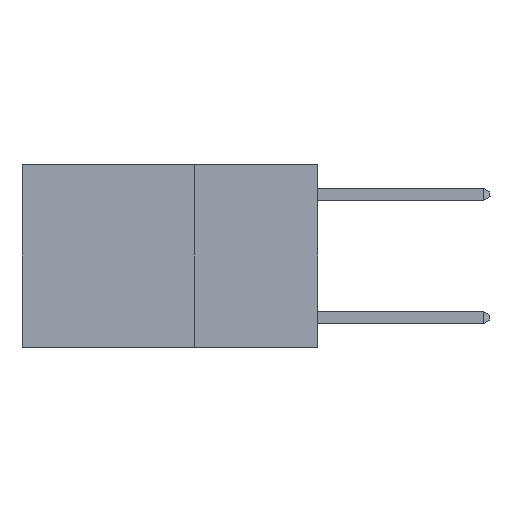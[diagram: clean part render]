
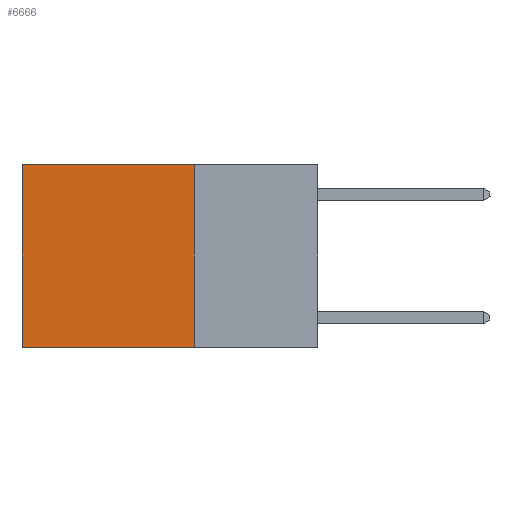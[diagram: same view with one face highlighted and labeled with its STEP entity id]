
A CAD part, left-side view. The second image highlights one B-rep face of the part: STEP entity #6666.
In plain terms, the highlighted planar face has unit normal (-1, 0, 0).
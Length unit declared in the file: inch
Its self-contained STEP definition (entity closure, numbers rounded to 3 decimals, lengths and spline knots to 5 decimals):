
#263 = AXIS2_PLACEMENT_3D ( 'NONE', #1253, #10188, #3912 ) ;
#319 = EDGE_CURVE ( 'NONE', #4889, #12411, #10377, .T. ) ;
#1130 = EDGE_CURVE ( 'NONE', #3066, #12411, #10007, .T. ) ;
#1253 = CARTESIAN_POINT ( 'NONE',  ( 0.2625, 0.25, 0. ) ) ;
#2576 = PLANE ( 'NONE',  #263 ) ;
#2891 = VECTOR ( 'NONE', #3564, 39.37008 ) ;
#3066 = VERTEX_POINT ( 'NONE', #11865 ) ;
#3209 = VECTOR ( 'NONE', #14238, 39.37008 ) ;
#3564 = DIRECTION ( 'NONE',  ( 0., 1., 0. ) ) ;
#3667 = ORIENTED_EDGE ( 'NONE', *, *, #1130, .F. ) ;
#3912 = DIRECTION ( 'NONE',  ( 0., 0., -1. ) ) ;
#4073 = ORIENTED_EDGE ( 'NONE', *, *, #15013, .F. ) ;
#4889 = VERTEX_POINT ( 'NONE', #7036 ) ;
#5493 = DIRECTION ( 'NONE',  ( 0., 0., -1. ) ) ;
#6666 = ADVANCED_FACE ( 'NONE', ( #12484 ), #2576, .F. ) ;
#6697 = VECTOR ( 'NONE', #9883, 39.37008 ) ;
#6782 = CARTESIAN_POINT ( 'NONE',  ( 0.2625, 0.25, 0. ) ) ;
#7036 = CARTESIAN_POINT ( 'NONE',  ( 0.2625, 0.6, 0. ) ) ;
#7069 = EDGE_CURVE ( 'NONE', #15027, #4889, #12113, .T. ) ;
#7765 = VECTOR ( 'NONE', #5493, 39.37008 ) ;
#8125 = CARTESIAN_POINT ( 'NONE',  ( 0.2625, 0.25, 0. ) ) ;
#9883 = DIRECTION ( 'NONE',  ( 0., 1., 0. ) ) ;
#10007 = LINE ( 'NONE', #12335, #6697 ) ;
#10188 = DIRECTION ( 'NONE',  ( 1., 0., 0. ) ) ;
#10322 = EDGE_LOOP ( 'NONE', ( #13167, #3667, #4073, #10782 ) ) ;
#10377 = LINE ( 'NONE', #12431, #3209 ) ;
#10782 = ORIENTED_EDGE ( 'NONE', *, *, #7069, .T. ) ;
#10975 = LINE ( 'NONE', #6782, #7765 ) ;
#11095 = CARTESIAN_POINT ( 'NONE',  ( 0.2625, 0.25, 0. ) ) ;
#11513 = CARTESIAN_POINT ( 'NONE',  ( 0.2625, 0.6, -0.37 ) ) ;
#11865 = CARTESIAN_POINT ( 'NONE',  ( 0.2625, 0.25, -0.37 ) ) ;
#12113 = LINE ( 'NONE', #11095, #2891 ) ;
#12335 = CARTESIAN_POINT ( 'NONE',  ( 0.2625, 0.25, -0.37 ) ) ;
#12411 = VERTEX_POINT ( 'NONE', #11513 ) ;
#12431 = CARTESIAN_POINT ( 'NONE',  ( 0.2625, 0.6, 0. ) ) ;
#12484 = FACE_OUTER_BOUND ( 'NONE', #10322, .T. ) ;
#13167 = ORIENTED_EDGE ( 'NONE', *, *, #319, .T. ) ;
#14238 = DIRECTION ( 'NONE',  ( 0., 0., -1. ) ) ;
#15013 = EDGE_CURVE ( 'NONE', #15027, #3066, #10975, .T. ) ;
#15027 = VERTEX_POINT ( 'NONE', #8125 ) ;
